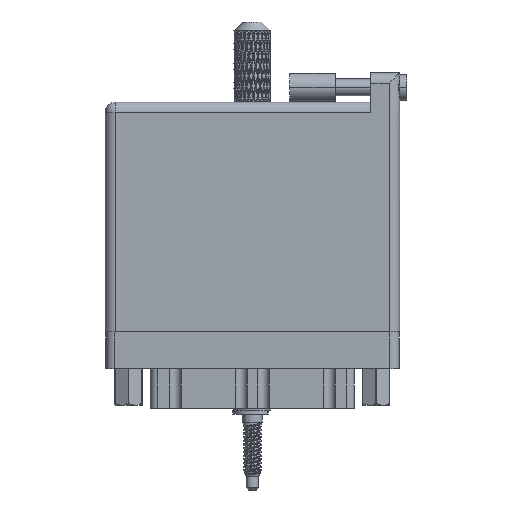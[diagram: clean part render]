
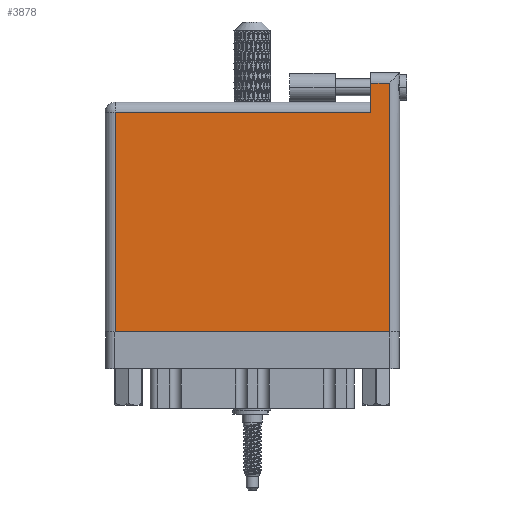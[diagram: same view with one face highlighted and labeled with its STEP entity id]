
A CAD part, front view. The second image highlights one B-rep face of the part: STEP entity #3878.
In plain terms, the highlighted face is planar.
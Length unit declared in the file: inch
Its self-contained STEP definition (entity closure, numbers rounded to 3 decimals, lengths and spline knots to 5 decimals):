
#740 = VERTEX_POINT ( 'NONE', #81251 ) ;
#2147 = CARTESIAN_POINT ( 'NONE',  ( 0., 0., 0. ) ) ;
#3181 = EDGE_CURVE ( 'NONE', #23080, #23755, #65910, .T. ) ;
#3727 = EDGE_CURVE ( 'NONE', #23755, #106049, #13174, .T. ) ;
#3878 = ADVANCED_FACE ( 'NONE', ( #80534 ), #47352, .F. ) ;
#10001 = ORIENTED_EDGE ( 'NONE', *, *, #97463, .T. ) ;
#10016 = DIRECTION ( 'NONE',  ( 0., -1., 0. ) ) ;
#10785 = CARTESIAN_POINT ( 'NONE',  ( 0., 1.566, 0. ) ) ;
#11930 = DIRECTION ( 'NONE',  ( 0., 0., -1. ) ) ;
#13174 = LINE ( 'NONE', #110322, #46402 ) ;
#13228 = DIRECTION ( 'NONE',  ( -1., 0., 0. ) ) ;
#14427 = DIRECTION ( 'NONE',  ( -1., 0., 0. ) ) ;
#17468 = CARTESIAN_POINT ( 'NONE',  ( 1.938, 0., 0. ) ) ;
#20112 = ORIENTED_EDGE ( 'NONE', *, *, #3181, .T. ) ;
#21800 = LINE ( 'NONE', #40092, #106824 ) ;
#22172 = ORIENTED_EDGE ( 'NONE', *, *, #27190, .T. ) ;
#23080 = VERTEX_POINT ( 'NONE', #72312 ) ;
#23755 = VERTEX_POINT ( 'NONE', #47701 ) ;
#24335 = ORIENTED_EDGE ( 'NONE', *, *, #36542, .T. ) ;
#27190 = EDGE_CURVE ( 'NONE', #740, #27260, #107888, .T. ) ;
#27260 = VERTEX_POINT ( 'NONE', #17468 ) ;
#36542 = EDGE_CURVE ( 'NONE', #40895, #740, #96369, .T. ) ;
#37295 = ORIENTED_EDGE ( 'NONE', *, *, #80512, .T. ) ;
#39826 = LINE ( 'NONE', #108985, #96531 ) ;
#40092 = CARTESIAN_POINT ( 'NONE',  ( 0., 1.496, 0. ) ) ;
#40895 = VERTEX_POINT ( 'NONE', #68679 ) ;
#43788 = CARTESIAN_POINT ( 'NONE',  ( 0.07, 0., 0. ) ) ;
#46402 = VECTOR ( 'NONE', #82930, 39.37008 ) ;
#47352 = PLANE ( 'NONE',  #110297 ) ;
#47701 = CARTESIAN_POINT ( 'NONE',  ( 1.811, 1.696, 0. ) ) ;
#52998 = ORIENTED_EDGE ( 'NONE', *, *, #3727, .T. ) ;
#60879 = VECTOR ( 'NONE', #10016, 39.37008 ) ;
#65910 = LINE ( 'NONE', #111596, #101344 ) ;
#68679 = CARTESIAN_POINT ( 'NONE',  ( 0.07, 1.496, 0. ) ) ;
#71953 = DIRECTION ( 'NONE',  ( -1., 0., 0. ) ) ;
#72312 = CARTESIAN_POINT ( 'NONE',  ( 1.938, 1.696, 0. ) ) ;
#80512 = EDGE_CURVE ( 'NONE', #27260, #23080, #39826, .T. ) ;
#80534 = FACE_OUTER_BOUND ( 'NONE', #94165, .T. ) ;
#81251 = CARTESIAN_POINT ( 'NONE',  ( 0.07, 0., 0. ) ) ;
#82154 = DIRECTION ( 'NONE',  ( 0., 1., 0. ) ) ;
#82930 = DIRECTION ( 'NONE',  ( 0., -1., 0. ) ) ;
#94165 = EDGE_LOOP ( 'NONE', ( #22172, #37295, #20112, #52998, #10001, #24335 ) ) ;
#94241 = VECTOR ( 'NONE', #109002, 39.37008 ) ;
#96369 = LINE ( 'NONE', #43788, #60879 ) ;
#96531 = VECTOR ( 'NONE', #82154, 39.37008 ) ;
#97463 = EDGE_CURVE ( 'NONE', #106049, #40895, #21800, .T. ) ;
#97542 = CARTESIAN_POINT ( 'NONE',  ( 1.811, 1.496, 0. ) ) ;
#101344 = VECTOR ( 'NONE', #14427, 39.37008 ) ;
#106049 = VERTEX_POINT ( 'NONE', #97542 ) ;
#106824 = VECTOR ( 'NONE', #13228, 39.37008 ) ;
#107888 = LINE ( 'NONE', #2147, #94241 ) ;
#108985 = CARTESIAN_POINT ( 'NONE',  ( 1.938, 1.766, 0. ) ) ;
#109002 = DIRECTION ( 'NONE',  ( 1., 0., 0. ) ) ;
#110297 = AXIS2_PLACEMENT_3D ( 'NONE', #10785, #11930, #71953 ) ;
#110322 = CARTESIAN_POINT ( 'NONE',  ( 1.811, 1.766, 0. ) ) ;
#111596 = CARTESIAN_POINT ( 'NONE',  ( 0., 1.696, 0. ) ) ;
